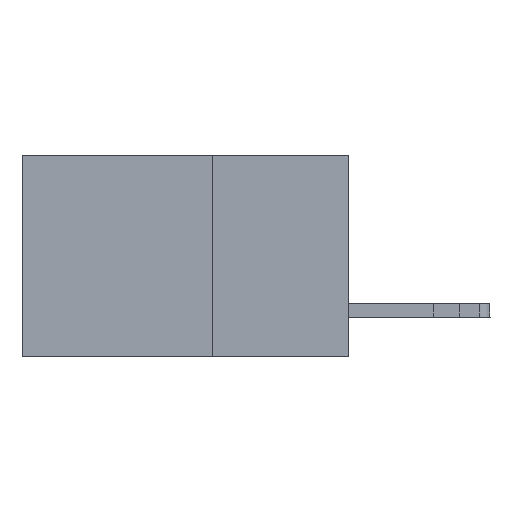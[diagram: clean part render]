
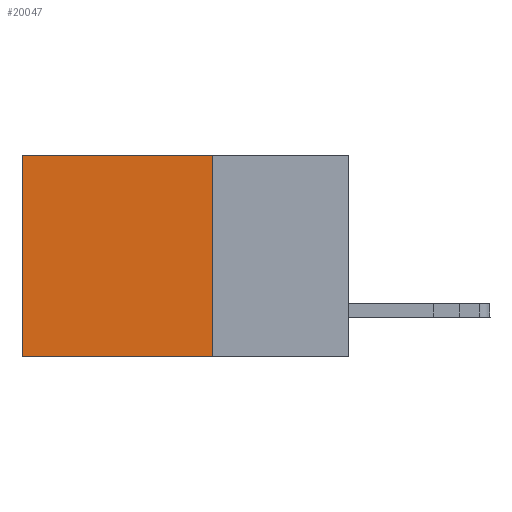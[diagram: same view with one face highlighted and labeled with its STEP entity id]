
A CAD part, left-side view. The second image highlights one B-rep face of the part: STEP entity #20047.
In plain terms, the highlighted planar face has unit normal (-1, 0, 0).
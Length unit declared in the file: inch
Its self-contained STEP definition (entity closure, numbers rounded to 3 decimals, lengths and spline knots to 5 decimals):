
#1620 = PLANE ( 'NONE',  #14063 ) ;
#2412 = ORIENTED_EDGE ( 'NONE', *, *, #18130, .F. ) ;
#2729 = CARTESIAN_POINT ( 'NONE',  ( 0.298, 0.25, 0. ) ) ;
#3091 = LINE ( 'NONE', #18470, #18536 ) ;
#3111 = VECTOR ( 'NONE', #23271, 39.37008 ) ;
#4607 = VERTEX_POINT ( 'NONE', #5462 ) ;
#4699 = CARTESIAN_POINT ( 'NONE',  ( 0.298, 0.25, -0.37 ) ) ;
#4708 = ORIENTED_EDGE ( 'NONE', *, *, #15853, .T. ) ;
#5388 = DIRECTION ( 'NONE',  ( 0., 0., -1. ) ) ;
#5462 = CARTESIAN_POINT ( 'NONE',  ( 0.298, 0.6, -0.37 ) ) ;
#5894 = VERTEX_POINT ( 'NONE', #2729 ) ;
#6568 = DIRECTION ( 'NONE',  ( 0., 1., 0. ) ) ;
#7396 = CARTESIAN_POINT ( 'NONE',  ( 0.298, 0.25, -0.37 ) ) ;
#8029 = LINE ( 'NONE', #10478, #3111 ) ;
#8799 = ORIENTED_EDGE ( 'NONE', *, *, #13012, .T. ) ;
#10478 = CARTESIAN_POINT ( 'NONE',  ( 0.298, 0.6, 0. ) ) ;
#11743 = VERTEX_POINT ( 'NONE', #15784 ) ;
#12363 = ORIENTED_EDGE ( 'NONE', *, *, #16934, .F. ) ;
#12376 = LINE ( 'NONE', #22985, #21540 ) ;
#13012 = EDGE_CURVE ( 'NONE', #5894, #11743, #12376, .T. ) ;
#14063 = AXIS2_PLACEMENT_3D ( 'NONE', #23618, #16297, #5388 ) ;
#15784 = CARTESIAN_POINT ( 'NONE',  ( 0.298, 0.6, 0. ) ) ;
#15853 = EDGE_CURVE ( 'NONE', #11743, #4607, #8029, .T. ) ;
#16297 = DIRECTION ( 'NONE',  ( 1., 0., 0. ) ) ;
#16934 = EDGE_CURVE ( 'NONE', #5894, #17233, #3091, .T. ) ;
#17233 = VERTEX_POINT ( 'NONE', #4699 ) ;
#18130 = EDGE_CURVE ( 'NONE', #17233, #4607, #19966, .T. ) ;
#18470 = CARTESIAN_POINT ( 'NONE',  ( 0.298, 0.25, 0. ) ) ;
#18536 = VECTOR ( 'NONE', #20499, 39.37008 ) ;
#18993 = FACE_OUTER_BOUND ( 'NONE', #19624, .T. ) ;
#19372 = VECTOR ( 'NONE', #22051, 39.37008 ) ;
#19624 = EDGE_LOOP ( 'NONE', ( #4708, #2412, #12363, #8799 ) ) ;
#19966 = LINE ( 'NONE', #7396, #19372 ) ;
#20047 = ADVANCED_FACE ( 'NONE', ( #18993 ), #1620, .F. ) ;
#20499 = DIRECTION ( 'NONE',  ( 0., 0., -1. ) ) ;
#21540 = VECTOR ( 'NONE', #6568, 39.37008 ) ;
#22051 = DIRECTION ( 'NONE',  ( 0., 1., 0. ) ) ;
#22985 = CARTESIAN_POINT ( 'NONE',  ( 0.298, 0.25, 0. ) ) ;
#23271 = DIRECTION ( 'NONE',  ( 0., 0., -1. ) ) ;
#23618 = CARTESIAN_POINT ( 'NONE',  ( 0.298, 0.25, 0. ) ) ;
